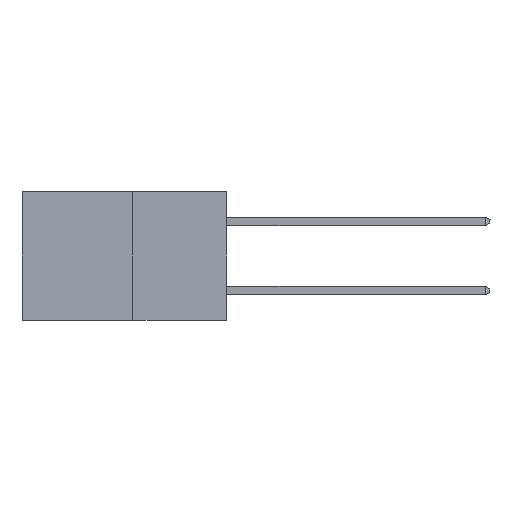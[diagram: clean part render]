
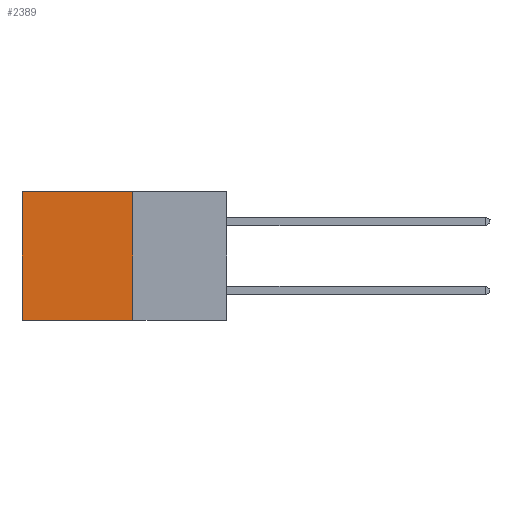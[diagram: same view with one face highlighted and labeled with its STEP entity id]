
A CAD part, left-side view. The second image highlights one B-rep face of the part: STEP entity #2389.
In plain terms, the highlighted planar face has unit normal (-1, 0, 0).
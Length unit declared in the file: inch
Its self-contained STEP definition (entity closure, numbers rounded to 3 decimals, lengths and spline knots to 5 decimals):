
#304 = VERTEX_POINT ( 'NONE', #7790 ) ;
#376 = CARTESIAN_POINT ( 'NONE',  ( 0.277, 0.27, 0. ) ) ;
#665 = ORIENTED_EDGE ( 'NONE', *, *, #15722, .F. ) ;
#766 = ORIENTED_EDGE ( 'NONE', *, *, #13706, .F. ) ;
#1099 = ORIENTED_EDGE ( 'NONE', *, *, #5646, .T. ) ;
#2014 = VERTEX_POINT ( 'NONE', #376 ) ;
#2389 = ADVANCED_FACE ( 'NONE', ( #5246 ), #14041, .F. ) ;
#2672 = VECTOR ( 'NONE', #18330, 39.37008 ) ;
#3733 = VECTOR ( 'NONE', #8782, 39.37008 ) ;
#3929 = VECTOR ( 'NONE', #11537, 39.37008 ) ;
#4190 = LINE ( 'NONE', #8804, #3733 ) ;
#4473 = CARTESIAN_POINT ( 'NONE',  ( 0.277, 0.59, 0. ) ) ;
#5246 = FACE_OUTER_BOUND ( 'NONE', #5536, .T. ) ;
#5536 = EDGE_LOOP ( 'NONE', ( #7149, #665, #766, #1099 ) ) ;
#5646 = EDGE_CURVE ( 'NONE', #2014, #14607, #4190, .T. ) ;
#5759 = CARTESIAN_POINT ( 'NONE',  ( 0.277, 0.59, -0.37 ) ) ;
#6265 = EDGE_CURVE ( 'NONE', #14607, #12420, #8515, .T. ) ;
#7149 = ORIENTED_EDGE ( 'NONE', *, *, #6265, .T. ) ;
#7790 = CARTESIAN_POINT ( 'NONE',  ( 0.277, 0.27, -0.37 ) ) ;
#8410 = CARTESIAN_POINT ( 'NONE',  ( 0.277, 0.27, -0.37 ) ) ;
#8515 = LINE ( 'NONE', #5759, #3929 ) ;
#8749 = DIRECTION ( 'NONE',  ( 0., 1., 0. ) ) ;
#8782 = DIRECTION ( 'NONE',  ( 0., 1., 0. ) ) ;
#8804 = CARTESIAN_POINT ( 'NONE',  ( 0.277, 0.27, 0. ) ) ;
#10257 = LINE ( 'NONE', #18195, #2672 ) ;
#11537 = DIRECTION ( 'NONE',  ( 0., 0., -1. ) ) ;
#12259 = CARTESIAN_POINT ( 'NONE',  ( 0.277, 0.27, -0.37 ) ) ;
#12420 = VERTEX_POINT ( 'NONE', #15261 ) ;
#13047 = VECTOR ( 'NONE', #8749, 39.37008 ) ;
#13706 = EDGE_CURVE ( 'NONE', #2014, #304, #10257, .T. ) ;
#13989 = LINE ( 'NONE', #8410, #13047 ) ;
#14041 = PLANE ( 'NONE',  #17992 ) ;
#14152 = DIRECTION ( 'NONE',  ( 0., 0., -1. ) ) ;
#14607 = VERTEX_POINT ( 'NONE', #4473 ) ;
#15058 = DIRECTION ( 'NONE',  ( 1., 0., 0. ) ) ;
#15261 = CARTESIAN_POINT ( 'NONE',  ( 0.277, 0.59, -0.37 ) ) ;
#15722 = EDGE_CURVE ( 'NONE', #304, #12420, #13989, .T. ) ;
#17992 = AXIS2_PLACEMENT_3D ( 'NONE', #12259, #15058, #14152 ) ;
#18195 = CARTESIAN_POINT ( 'NONE',  ( 0.277, 0.27, -0.37 ) ) ;
#18330 = DIRECTION ( 'NONE',  ( 0., 0., -1. ) ) ;
